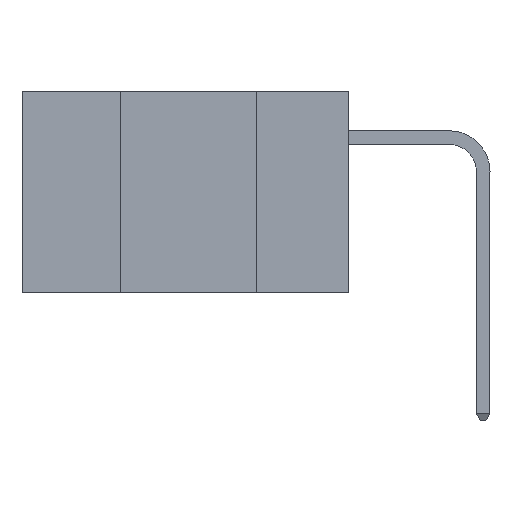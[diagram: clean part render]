
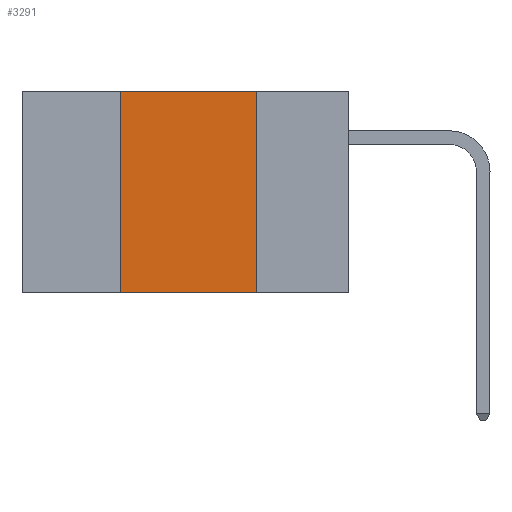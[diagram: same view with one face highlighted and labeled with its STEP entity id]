
A CAD part, left-side view. The second image highlights one B-rep face of the part: STEP entity #3291.
In plain terms, the highlighted planar face has unit normal (-1, 0, 0).
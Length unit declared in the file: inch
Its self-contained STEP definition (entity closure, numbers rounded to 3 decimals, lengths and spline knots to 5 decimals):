
#75 = EDGE_CURVE ( 'NONE', #5868, #3681, #2242, .T. ) ;
#590 = CARTESIAN_POINT ( 'NONE',  ( 0., 0.6, 0. ) ) ;
#1172 = VECTOR ( 'NONE', #5457, 39.37008 ) ;
#1586 = PLANE ( 'NONE',  #6559 ) ;
#2242 = LINE ( 'NONE', #11514, #5751 ) ;
#2434 = EDGE_CURVE ( 'NONE', #7359, #3681, #3004, .T. ) ;
#2497 = EDGE_LOOP ( 'NONE', ( #8425, #4523, #3786, #8986 ) ) ;
#2555 = EDGE_CURVE ( 'NONE', #7359, #5114, #11681, .T. ) ;
#3004 = LINE ( 'NONE', #10740, #1172 ) ;
#3291 = ADVANCED_FACE ( 'NONE', ( #4793 ), #1586, .F. ) ;
#3327 = LINE ( 'NONE', #8231, #5182 ) ;
#3681 = VERTEX_POINT ( 'NONE', #11940 ) ;
#3786 = ORIENTED_EDGE ( 'NONE', *, *, #2555, .F. ) ;
#4173 = DIRECTION ( 'NONE',  ( 0., 0., -1. ) ) ;
#4523 = ORIENTED_EDGE ( 'NONE', *, *, #8760, .F. ) ;
#4793 = FACE_OUTER_BOUND ( 'NONE', #2497, .T. ) ;
#4953 = CARTESIAN_POINT ( 'NONE',  ( 0., 0.17, 0. ) ) ;
#4968 = DIRECTION ( 'NONE',  ( 0., -1., 0. ) ) ;
#5114 = VERTEX_POINT ( 'NONE', #6943 ) ;
#5182 = VECTOR ( 'NONE', #4968, 39.37008 ) ;
#5405 = CARTESIAN_POINT ( 'NONE',  ( 0., 0.42, -0.37 ) ) ;
#5457 = DIRECTION ( 'NONE',  ( 0., -1., 0. ) ) ;
#5751 = VECTOR ( 'NONE', #4173, 39.37008 ) ;
#5786 = CARTESIAN_POINT ( 'NONE',  ( 0., 0.42, 0. ) ) ;
#5826 = VECTOR ( 'NONE', #11151, 39.37008 ) ;
#5868 = VERTEX_POINT ( 'NONE', #4953 ) ;
#6559 = AXIS2_PLACEMENT_3D ( 'NONE', #590, #10182, #13214 ) ;
#6943 = CARTESIAN_POINT ( 'NONE',  ( 0., 0.42, 0. ) ) ;
#7359 = VERTEX_POINT ( 'NONE', #5405 ) ;
#8231 = CARTESIAN_POINT ( 'NONE',  ( 0., 0.6, 0. ) ) ;
#8425 = ORIENTED_EDGE ( 'NONE', *, *, #75, .F. ) ;
#8760 = EDGE_CURVE ( 'NONE', #5114, #5868, #3327, .T. ) ;
#8986 = ORIENTED_EDGE ( 'NONE', *, *, #2434, .T. ) ;
#10182 = DIRECTION ( 'NONE',  ( 1., 0., 0. ) ) ;
#10740 = CARTESIAN_POINT ( 'NONE',  ( 0., 0.6, -0.37 ) ) ;
#11151 = DIRECTION ( 'NONE',  ( 0., 0., 1. ) ) ;
#11514 = CARTESIAN_POINT ( 'NONE',  ( 0., 0.17, 0. ) ) ;
#11681 = LINE ( 'NONE', #5786, #5826 ) ;
#11940 = CARTESIAN_POINT ( 'NONE',  ( 0., 0.17, -0.37 ) ) ;
#13214 = DIRECTION ( 'NONE',  ( 0., 0., -1. ) ) ;
